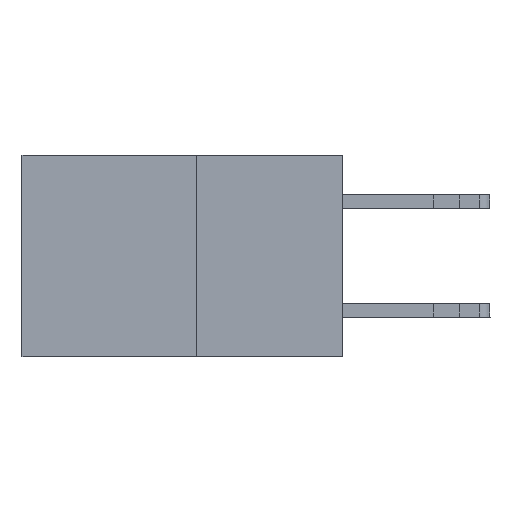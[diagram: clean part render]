
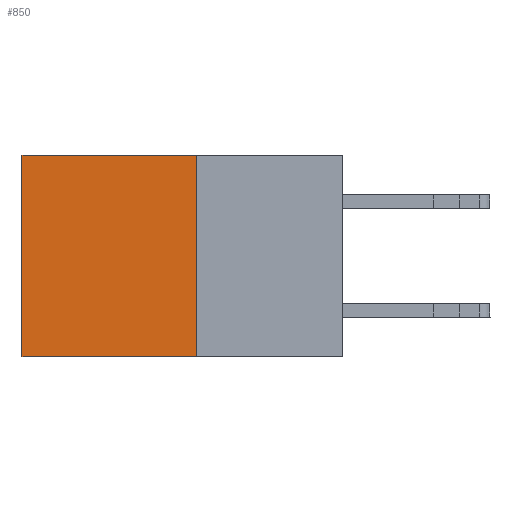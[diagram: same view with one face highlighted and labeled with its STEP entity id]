
A CAD part, left-side view. The second image highlights one B-rep face of the part: STEP entity #850.
In plain terms, the highlighted planar face has unit normal (-1, 0, 0).
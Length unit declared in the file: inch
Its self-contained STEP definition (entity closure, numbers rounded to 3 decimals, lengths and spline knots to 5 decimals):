
#129 = VECTOR ( 'NONE', #2738, 39.37008 ) ;
#850 = ADVANCED_FACE ( 'NONE', ( #9682 ), #13989, .F. ) ;
#1187 = CARTESIAN_POINT ( 'NONE',  ( 0.277, 0.27, -0.37 ) ) ;
#2738 = DIRECTION ( 'NONE',  ( 0., 0., -1. ) ) ;
#3266 = CARTESIAN_POINT ( 'NONE',  ( 0.277, 0.27, 0. ) ) ;
#3724 = ORIENTED_EDGE ( 'NONE', *, *, #10624, .F. ) ;
#4381 = EDGE_CURVE ( 'NONE', #7253, #21347, #14277, .T. ) ;
#4619 = CARTESIAN_POINT ( 'NONE',  ( 0.277, 0.59, -0.37 ) ) ;
#4734 = DIRECTION ( 'NONE',  ( 0., 1., 0. ) ) ;
#4855 = LINE ( 'NONE', #15028, #129 ) ;
#5189 = AXIS2_PLACEMENT_3D ( 'NONE', #8092, #16215, #19945 ) ;
#5703 = CARTESIAN_POINT ( 'NONE',  ( 0.277, 0.27, -0.37 ) ) ;
#5737 = LINE ( 'NONE', #1187, #19718 ) ;
#6276 = VECTOR ( 'NONE', #14479, 39.37008 ) ;
#7170 = ORIENTED_EDGE ( 'NONE', *, *, #12508, .T. ) ;
#7253 = VERTEX_POINT ( 'NONE', #3266 ) ;
#8092 = CARTESIAN_POINT ( 'NONE',  ( 0.277, 0.27, -0.37 ) ) ;
#9682 = FACE_OUTER_BOUND ( 'NONE', #16443, .T. ) ;
#10211 = EDGE_CURVE ( 'NONE', #7253, #19721, #5737, .T. ) ;
#10624 = EDGE_CURVE ( 'NONE', #19721, #11469, #20812, .T. ) ;
#11469 = VERTEX_POINT ( 'NONE', #4619 ) ;
#11732 = DIRECTION ( 'NONE',  ( 0., 0., -1. ) ) ;
#12508 = EDGE_CURVE ( 'NONE', #21347, #11469, #4855, .T. ) ;
#12955 = CARTESIAN_POINT ( 'NONE',  ( 0.277, 0.27, 0. ) ) ;
#13733 = VECTOR ( 'NONE', #4734, 39.37008 ) ;
#13989 = PLANE ( 'NONE',  #5189 ) ;
#14197 = ORIENTED_EDGE ( 'NONE', *, *, #4381, .T. ) ;
#14277 = LINE ( 'NONE', #12955, #13733 ) ;
#14479 = DIRECTION ( 'NONE',  ( 0., 1., 0. ) ) ;
#15028 = CARTESIAN_POINT ( 'NONE',  ( 0.277, 0.59, -0.37 ) ) ;
#16215 = DIRECTION ( 'NONE',  ( 1., 0., 0. ) ) ;
#16357 = ORIENTED_EDGE ( 'NONE', *, *, #10211, .F. ) ;
#16443 = EDGE_LOOP ( 'NONE', ( #7170, #3724, #16357, #14197 ) ) ;
#16907 = CARTESIAN_POINT ( 'NONE',  ( 0.277, 0.27, -0.37 ) ) ;
#18034 = CARTESIAN_POINT ( 'NONE',  ( 0.277, 0.59, 0. ) ) ;
#19718 = VECTOR ( 'NONE', #11732, 39.37008 ) ;
#19721 = VERTEX_POINT ( 'NONE', #16907 ) ;
#19945 = DIRECTION ( 'NONE',  ( 0., 0., -1. ) ) ;
#20812 = LINE ( 'NONE', #5703, #6276 ) ;
#21347 = VERTEX_POINT ( 'NONE', #18034 ) ;
